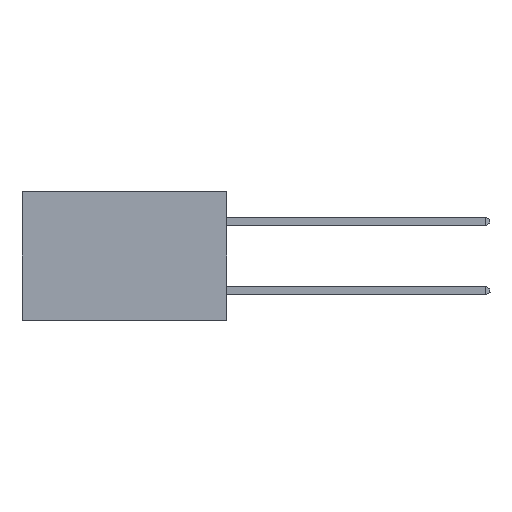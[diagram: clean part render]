
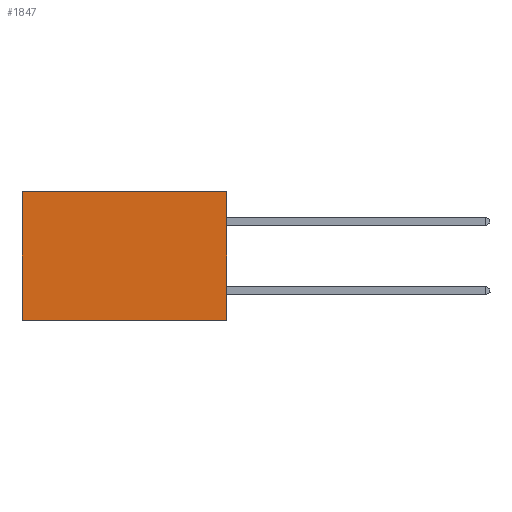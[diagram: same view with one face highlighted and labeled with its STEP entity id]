
A CAD part, left-side view. The second image highlights one B-rep face of the part: STEP entity #1847.
In plain terms, the highlighted planar face has unit normal (-1, 0, 0).
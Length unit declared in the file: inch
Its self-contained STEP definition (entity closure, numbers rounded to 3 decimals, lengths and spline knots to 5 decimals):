
#80 = VECTOR ( 'NONE', #3234, 39.37008 ) ;
#334 = VERTEX_POINT ( 'NONE', #4670 ) ;
#352 = VERTEX_POINT ( 'NONE', #5473 ) ;
#505 = CARTESIAN_POINT ( 'NONE',  ( 0.277, 0., 0. ) ) ;
#1248 = VECTOR ( 'NONE', #2669, 39.37008 ) ;
#1453 = ORIENTED_EDGE ( 'NONE', *, *, #4504, .T. ) ;
#1617 = ORIENTED_EDGE ( 'NONE', *, *, #5126, .F. ) ;
#1638 = FACE_OUTER_BOUND ( 'NONE', #4012, .T. ) ;
#1643 = EDGE_CURVE ( 'NONE', #2653, #2915, #3641, .T. ) ;
#1740 = VECTOR ( 'NONE', #7574, 39.37008 ) ;
#1847 = ADVANCED_FACE ( 'NONE', ( #1638 ), #4840, .F. ) ;
#2580 = LINE ( 'NONE', #3247, #80 ) ;
#2620 = ORIENTED_EDGE ( 'NONE', *, *, #1643, .T. ) ;
#2653 = VERTEX_POINT ( 'NONE', #505 ) ;
#2669 = DIRECTION ( 'NONE',  ( 0., 0., -1. ) ) ;
#2717 = CARTESIAN_POINT ( 'NONE',  ( 0.277, 0.59, -0.37 ) ) ;
#2915 = VERTEX_POINT ( 'NONE', #6849 ) ;
#3064 = LINE ( 'NONE', #2717, #1248 ) ;
#3089 = ORIENTED_EDGE ( 'NONE', *, *, #4316, .F. ) ;
#3234 = DIRECTION ( 'NONE',  ( 0., 0., -1. ) ) ;
#3247 = CARTESIAN_POINT ( 'NONE',  ( 0.277, 0., -0.37 ) ) ;
#3309 = DIRECTION ( 'NONE',  ( 0., 1., 0. ) ) ;
#3641 = LINE ( 'NONE', #4862, #6311 ) ;
#3761 = CARTESIAN_POINT ( 'NONE',  ( 0.277, 0., -0.37 ) ) ;
#3863 = DIRECTION ( 'NONE',  ( 0., 0., -1. ) ) ;
#4012 = EDGE_LOOP ( 'NONE', ( #1453, #1617, #3089, #2620 ) ) ;
#4316 = EDGE_CURVE ( 'NONE', #2653, #352, #2580, .T. ) ;
#4504 = EDGE_CURVE ( 'NONE', #2915, #334, #3064, .T. ) ;
#4670 = CARTESIAN_POINT ( 'NONE',  ( 0.277, 0.59, -0.37 ) ) ;
#4840 = PLANE ( 'NONE',  #5792 ) ;
#4842 = LINE ( 'NONE', #6706, #1740 ) ;
#4862 = CARTESIAN_POINT ( 'NONE',  ( 0.277, 0., 0. ) ) ;
#5126 = EDGE_CURVE ( 'NONE', #352, #334, #4842, .T. ) ;
#5402 = DIRECTION ( 'NONE',  ( 1., 0., 0. ) ) ;
#5473 = CARTESIAN_POINT ( 'NONE',  ( 0.277, 0., -0.37 ) ) ;
#5792 = AXIS2_PLACEMENT_3D ( 'NONE', #3761, #5402, #3863 ) ;
#6311 = VECTOR ( 'NONE', #3309, 39.37008 ) ;
#6706 = CARTESIAN_POINT ( 'NONE',  ( 0.277, 0., -0.37 ) ) ;
#6849 = CARTESIAN_POINT ( 'NONE',  ( 0.277, 0.59, 0. ) ) ;
#7574 = DIRECTION ( 'NONE',  ( 0., 1., 0. ) ) ;
